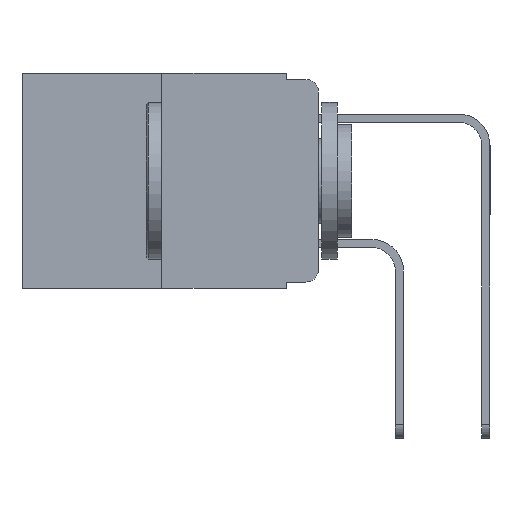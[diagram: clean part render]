
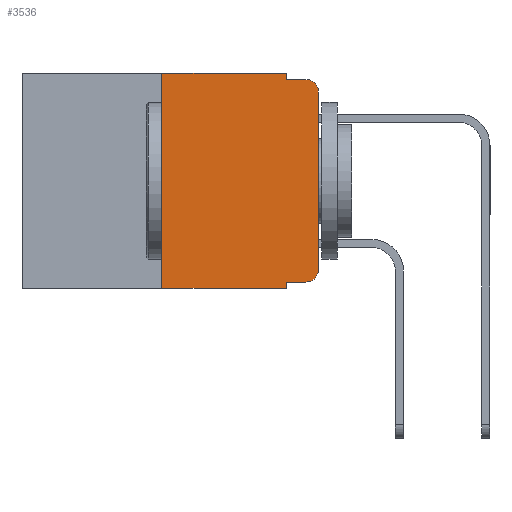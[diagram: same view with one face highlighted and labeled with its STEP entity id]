
A CAD part, left-side view. The second image highlights one B-rep face of the part: STEP entity #3536.
In plain terms, the highlighted planar face has unit normal (-1, 0, 0).
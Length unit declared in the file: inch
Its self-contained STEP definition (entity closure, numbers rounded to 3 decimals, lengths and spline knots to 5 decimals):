
#51 = AXIS2_PLACEMENT_3D ( 'NONE', #13796, #6428, #19434 ) ;
#71 = CARTESIAN_POINT ( 'NONE',  ( 0., 0.051, -0.343 ) ) ;
#1184 = LINE ( 'NONE', #1743, #5601 ) ;
#1364 = VECTOR ( 'NONE', #16618, 39.37008 ) ;
#1674 = CARTESIAN_POINT ( 'NONE',  ( 0., 0.473, 0. ) ) ;
#1743 = CARTESIAN_POINT ( 'NONE',  ( 0., 0.051, 0. ) ) ;
#1963 = LINE ( 'NONE', #15253, #2556 ) ;
#2044 = ORIENTED_EDGE ( 'NONE', *, *, #21759, .T. ) ;
#2336 = ORIENTED_EDGE ( 'NONE', *, *, #19451, .F. ) ;
#2556 = VECTOR ( 'NONE', #17066, 39.37008 ) ;
#2575 = CARTESIAN_POINT ( 'NONE',  ( 0., 0., -0.313 ) ) ;
#2702 = DIRECTION ( 'NONE',  ( -1., 0., 0. ) ) ;
#2727 = EDGE_CURVE ( 'NONE', #11200, #23729, #5183, .T. ) ;
#3402 = VERTEX_POINT ( 'NONE', #6014 ) ;
#3497 = EDGE_CURVE ( 'NONE', #14538, #20482, #23214, .T. ) ;
#3536 = ADVANCED_FACE ( 'NONE', ( #17704 ), #13873, .F. ) ;
#4644 = CARTESIAN_POINT ( 'NONE',  ( 0., 0.051, -0.333 ) ) ;
#5183 = LINE ( 'NONE', #16348, #14555 ) ;
#5489 = EDGE_CURVE ( 'NONE', #7125, #11200, #21393, .T. ) ;
#5558 = ORIENTED_EDGE ( 'NONE', *, *, #2727, .T. ) ;
#5601 = VECTOR ( 'NONE', #12987, 39.37008 ) ;
#5666 = VERTEX_POINT ( 'NONE', #11058 ) ;
#5848 = CARTESIAN_POINT ( 'NONE',  ( 0., 0.051, 0. ) ) ;
#5877 = ORIENTED_EDGE ( 'NONE', *, *, #3497, .F. ) ;
#6014 = CARTESIAN_POINT ( 'NONE',  ( 0., 0.051, -0.01 ) ) ;
#6428 = DIRECTION ( 'NONE',  ( 1., 0., 0. ) ) ;
#6985 = LINE ( 'NONE', #1674, #1364 ) ;
#7072 = ORIENTED_EDGE ( 'NONE', *, *, #11487, .F. ) ;
#7125 = VERTEX_POINT ( 'NONE', #22861 ) ;
#7340 = ORIENTED_EDGE ( 'NONE', *, *, #19598, .F. ) ;
#7652 = AXIS2_PLACEMENT_3D ( 'NONE', #8396, #21340, #10255 ) ;
#8153 = CARTESIAN_POINT ( 'NONE',  ( 0., 0.051, 0. ) ) ;
#8160 = CARTESIAN_POINT ( 'NONE',  ( 0., 0.25, 0. ) ) ;
#8338 = VECTOR ( 'NONE', #14634, 39.37008 ) ;
#8396 = CARTESIAN_POINT ( 'NONE',  ( 0., 0.02, -0.313 ) ) ;
#8528 = ORIENTED_EDGE ( 'NONE', *, *, #18759, .F. ) ;
#9496 = LINE ( 'NONE', #21955, #8338 ) ;
#9772 = VERTEX_POINT ( 'NONE', #5848 ) ;
#10020 = DIRECTION ( 'NONE',  ( 0., 0., 1. ) ) ;
#10255 = DIRECTION ( 'NONE',  ( 0., 0., -1. ) ) ;
#10680 = VECTOR ( 'NONE', #12164, 39.37008 ) ;
#11058 = CARTESIAN_POINT ( 'NONE',  ( 0., 0.051, -0.333 ) ) ;
#11121 = ORIENTED_EDGE ( 'NONE', *, *, #12799, .T. ) ;
#11185 = CARTESIAN_POINT ( 'NONE',  ( 0., 0., -0.03 ) ) ;
#11200 = VERTEX_POINT ( 'NONE', #2575 ) ;
#11487 = EDGE_CURVE ( 'NONE', #5666, #20022, #1184, .T. ) ;
#12164 = DIRECTION ( 'NONE',  ( 0., -1., 0. ) ) ;
#12216 = VERTEX_POINT ( 'NONE', #17564 ) ;
#12799 = EDGE_CURVE ( 'NONE', #23729, #12216, #20941, .T. ) ;
#12813 = VECTOR ( 'NONE', #10020, 39.37008 ) ;
#12987 = DIRECTION ( 'NONE',  ( 0., 0., -1. ) ) ;
#13796 = CARTESIAN_POINT ( 'NONE',  ( 0., 0.473, 0. ) ) ;
#13873 = PLANE ( 'NONE',  #51 ) ;
#13932 = CARTESIAN_POINT ( 'NONE',  ( 0., 0.02, -0.03 ) ) ;
#14538 = VERTEX_POINT ( 'NONE', #20859 ) ;
#14555 = VECTOR ( 'NONE', #17193, 39.37008 ) ;
#14634 = DIRECTION ( 'NONE',  ( 0., -1., 0. ) ) ;
#15253 = CARTESIAN_POINT ( 'NONE',  ( 0., 0.051, -0.01 ) ) ;
#15647 = LINE ( 'NONE', #4644, #10680 ) ;
#15785 = DIRECTION ( 'NONE',  ( 0., 0., -1. ) ) ;
#16307 = CARTESIAN_POINT ( 'NONE',  ( 0., 0.25, 0. ) ) ;
#16348 = CARTESIAN_POINT ( 'NONE',  ( 0., 0., 0. ) ) ;
#16618 = DIRECTION ( 'NONE',  ( 0., -1., 0. ) ) ;
#17066 = DIRECTION ( 'NONE',  ( 0., -1., 0. ) ) ;
#17134 = VECTOR ( 'NONE', #22971, 39.37008 ) ;
#17193 = DIRECTION ( 'NONE',  ( 0., 0., 1. ) ) ;
#17464 = AXIS2_PLACEMENT_3D ( 'NONE', #13932, #2702, #15785 ) ;
#17523 = ORIENTED_EDGE ( 'NONE', *, *, #24046, .T. ) ;
#17564 = CARTESIAN_POINT ( 'NONE',  ( 0., 0.02, -0.01 ) ) ;
#17704 = FACE_OUTER_BOUND ( 'NONE', #22333, .T. ) ;
#18695 = ORIENTED_EDGE ( 'NONE', *, *, #5489, .T. ) ;
#18759 = EDGE_CURVE ( 'NONE', #20482, #9772, #6985, .T. ) ;
#19434 = DIRECTION ( 'NONE',  ( 0., 0., -1. ) ) ;
#19451 = EDGE_CURVE ( 'NONE', #3402, #12216, #1963, .T. ) ;
#19598 = EDGE_CURVE ( 'NONE', #9772, #3402, #22643, .T. ) ;
#20022 = VERTEX_POINT ( 'NONE', #71 ) ;
#20482 = VERTEX_POINT ( 'NONE', #16307 ) ;
#20859 = CARTESIAN_POINT ( 'NONE',  ( 0., 0.25, -0.343 ) ) ;
#20941 = CIRCLE ( 'NONE', #17464, 0.02 ) ;
#21340 = DIRECTION ( 'NONE',  ( -1., 0., 0. ) ) ;
#21393 = CIRCLE ( 'NONE', #7652, 0.02 ) ;
#21759 = EDGE_CURVE ( 'NONE', #14538, #20022, #9496, .T. ) ;
#21955 = CARTESIAN_POINT ( 'NONE',  ( 0., 0.473, -0.343 ) ) ;
#22333 = EDGE_LOOP ( 'NONE', ( #5558, #11121, #2336, #7340, #8528, #5877, #2044, #7072, #17523, #18695 ) ) ;
#22643 = LINE ( 'NONE', #8153, #17134 ) ;
#22861 = CARTESIAN_POINT ( 'NONE',  ( 0., 0.02, -0.333 ) ) ;
#22971 = DIRECTION ( 'NONE',  ( 0., 0., -1. ) ) ;
#23214 = LINE ( 'NONE', #8160, #12813 ) ;
#23729 = VERTEX_POINT ( 'NONE', #11185 ) ;
#24046 = EDGE_CURVE ( 'NONE', #5666, #7125, #15647, .T. ) ;
